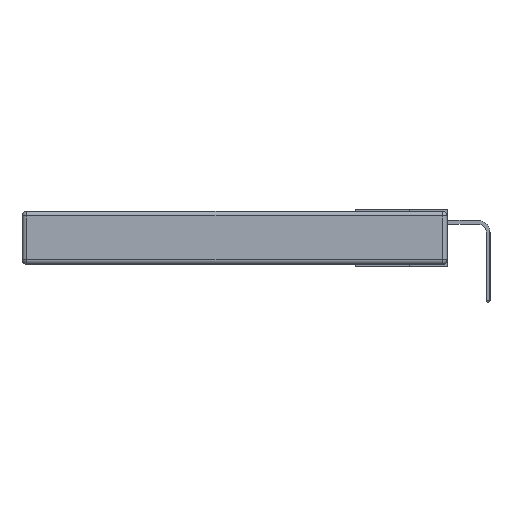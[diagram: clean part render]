
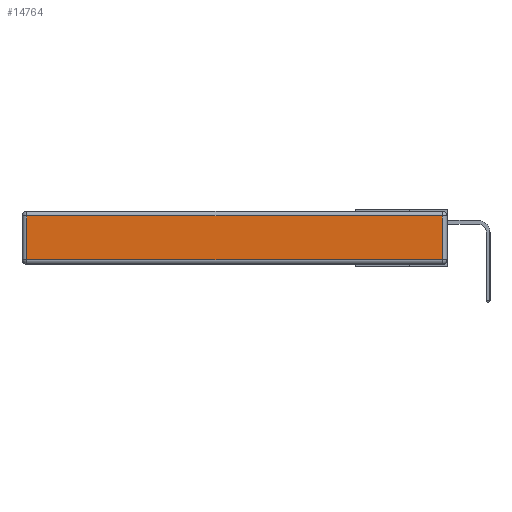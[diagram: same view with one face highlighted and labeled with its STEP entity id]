
A CAD part, left-side view. The second image highlights one B-rep face of the part: STEP entity #14764.
In plain terms, the highlighted planar face has unit normal (-1, 0, 0).
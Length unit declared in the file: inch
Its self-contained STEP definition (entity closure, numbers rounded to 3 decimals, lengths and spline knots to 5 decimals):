
#367 = LINE ( 'NONE', #16683, #14793 ) ;
#504 = CARTESIAN_POINT ( 'NONE',  ( 0., 2.72, -0.03 ) ) ;
#956 = EDGE_LOOP ( 'NONE', ( #16463, #2740, #15052, #8838 ) ) ;
#1487 = CARTESIAN_POINT ( 'NONE',  ( 0., 0., -0.343 ) ) ;
#2208 = LINE ( 'NONE', #6412, #12187 ) ;
#2349 = EDGE_CURVE ( 'NONE', #6090, #5059, #15193, .T. ) ;
#2740 = ORIENTED_EDGE ( 'NONE', *, *, #7841, .T. ) ;
#4419 = FACE_OUTER_BOUND ( 'NONE', #956, .T. ) ;
#5059 = VERTEX_POINT ( 'NONE', #12091 ) ;
#5644 = VECTOR ( 'NONE', #10849, 39.37008 ) ;
#5751 = CARTESIAN_POINT ( 'NONE',  ( 0., 0., -0.313 ) ) ;
#6066 = DIRECTION ( 'NONE',  ( 0., 0., -1. ) ) ;
#6090 = VERTEX_POINT ( 'NONE', #6882 ) ;
#6412 = CARTESIAN_POINT ( 'NONE',  ( 0., 2.72, -0.343 ) ) ;
#6882 = CARTESIAN_POINT ( 'NONE',  ( 0., 2.72, -0.313 ) ) ;
#7268 = EDGE_CURVE ( 'NONE', #11146, #6090, #2208, .T. ) ;
#7841 = EDGE_CURVE ( 'NONE', #5059, #16379, #367, .T. ) ;
#8046 = DIRECTION ( 'NONE',  ( 0., 0., 1. ) ) ;
#8727 = CARTESIAN_POINT ( 'NONE',  ( 0., 0.03, -0.03 ) ) ;
#8838 = ORIENTED_EDGE ( 'NONE', *, *, #7268, .T. ) ;
#8910 = CARTESIAN_POINT ( 'NONE',  ( 0., 2.75, -0.03 ) ) ;
#9020 = LINE ( 'NONE', #8910, #15969 ) ;
#9150 = AXIS2_PLACEMENT_3D ( 'NONE', #1487, #15671, #8046 ) ;
#10849 = DIRECTION ( 'NONE',  ( 0., -1., 0. ) ) ;
#11146 = VERTEX_POINT ( 'NONE', #504 ) ;
#11792 = PLANE ( 'NONE',  #9150 ) ;
#12091 = CARTESIAN_POINT ( 'NONE',  ( 0., 0.03, -0.313 ) ) ;
#12187 = VECTOR ( 'NONE', #6066, 39.37008 ) ;
#14124 = DIRECTION ( 'NONE',  ( 0., 1., 0. ) ) ;
#14764 = ADVANCED_FACE ( 'NONE', ( #4419 ), #11792, .T. ) ;
#14793 = VECTOR ( 'NONE', #15214, 39.37008 ) ;
#15052 = ORIENTED_EDGE ( 'NONE', *, *, #16800, .T. ) ;
#15193 = LINE ( 'NONE', #5751, #5644 ) ;
#15214 = DIRECTION ( 'NONE',  ( 0., 0., 1. ) ) ;
#15671 = DIRECTION ( 'NONE',  ( -1., 0., 0. ) ) ;
#15969 = VECTOR ( 'NONE', #14124, 39.37008 ) ;
#16379 = VERTEX_POINT ( 'NONE', #8727 ) ;
#16463 = ORIENTED_EDGE ( 'NONE', *, *, #2349, .T. ) ;
#16683 = CARTESIAN_POINT ( 'NONE',  ( 0., 0.03, -0.343 ) ) ;
#16800 = EDGE_CURVE ( 'NONE', #16379, #11146, #9020, .T. ) ;
